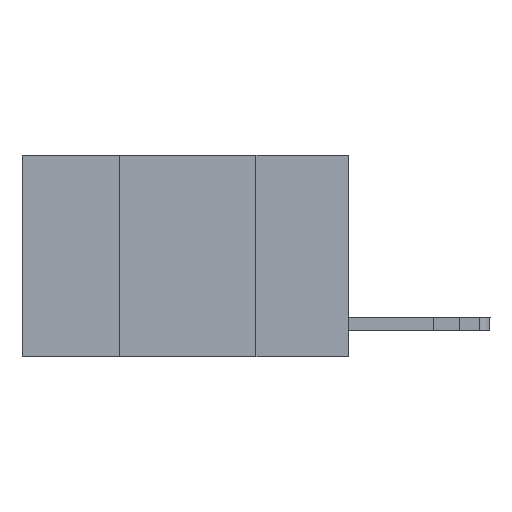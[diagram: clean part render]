
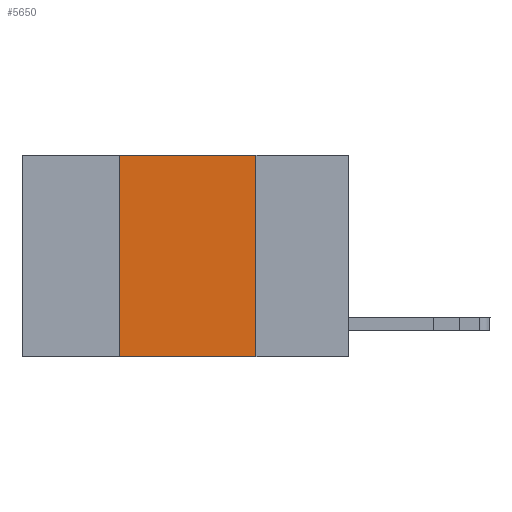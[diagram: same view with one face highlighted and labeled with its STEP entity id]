
A CAD part, left-side view. The second image highlights one B-rep face of the part: STEP entity #5650.
In plain terms, the highlighted planar face has unit normal (-1, 0, 0).
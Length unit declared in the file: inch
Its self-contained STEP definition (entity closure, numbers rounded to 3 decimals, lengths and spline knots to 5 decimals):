
#277 = VECTOR ( 'NONE', #6306, 39.37008 ) ;
#402 = CARTESIAN_POINT ( 'NONE',  ( 0., 0.17, 0. ) ) ;
#588 = VECTOR ( 'NONE', #5456, 39.37008 ) ;
#689 = AXIS2_PLACEMENT_3D ( 'NONE', #2539, #6544, #3451 ) ;
#714 = ORIENTED_EDGE ( 'NONE', *, *, #10044, .F. ) ;
#1664 = PLANE ( 'NONE',  #689 ) ;
#2024 = LINE ( 'NONE', #5980, #6707 ) ;
#2171 = EDGE_CURVE ( 'NONE', #4611, #5207, #12647, .T. ) ;
#2201 = DIRECTION ( 'NONE',  ( 0., -1., 0. ) ) ;
#2539 = CARTESIAN_POINT ( 'NONE',  ( 0., 0.6, 0. ) ) ;
#2913 = EDGE_LOOP ( 'NONE', ( #714, #7543, #7602, #7246 ) ) ;
#3346 = VERTEX_POINT ( 'NONE', #12955 ) ;
#3451 = DIRECTION ( 'NONE',  ( 0., 0., -1. ) ) ;
#4249 = CARTESIAN_POINT ( 'NONE',  ( 0., 0.42, 0. ) ) ;
#4342 = LINE ( 'NONE', #11333, #10923 ) ;
#4425 = CARTESIAN_POINT ( 'NONE',  ( 0., 0.17, -0.37 ) ) ;
#4611 = VERTEX_POINT ( 'NONE', #6180 ) ;
#5207 = VERTEX_POINT ( 'NONE', #4425 ) ;
#5456 = DIRECTION ( 'NONE',  ( 0., -1., 0. ) ) ;
#5650 = ADVANCED_FACE ( 'NONE', ( #12663 ), #1664, .F. ) ;
#5980 = CARTESIAN_POINT ( 'NONE',  ( 0., 0.17, 0. ) ) ;
#6180 = CARTESIAN_POINT ( 'NONE',  ( 0., 0.42, -0.37 ) ) ;
#6306 = DIRECTION ( 'NONE',  ( 0., 0., 1. ) ) ;
#6544 = DIRECTION ( 'NONE',  ( 1., 0., 0. ) ) ;
#6707 = VECTOR ( 'NONE', #12764, 39.37008 ) ;
#7242 = LINE ( 'NONE', #4249, #277 ) ;
#7246 = ORIENTED_EDGE ( 'NONE', *, *, #2171, .T. ) ;
#7300 = VERTEX_POINT ( 'NONE', #402 ) ;
#7543 = ORIENTED_EDGE ( 'NONE', *, *, #8030, .F. ) ;
#7602 = ORIENTED_EDGE ( 'NONE', *, *, #10203, .F. ) ;
#7717 = CARTESIAN_POINT ( 'NONE',  ( 0., 0.6, -0.37 ) ) ;
#8030 = EDGE_CURVE ( 'NONE', #3346, #7300, #4342, .T. ) ;
#10044 = EDGE_CURVE ( 'NONE', #7300, #5207, #2024, .T. ) ;
#10203 = EDGE_CURVE ( 'NONE', #4611, #3346, #7242, .T. ) ;
#10923 = VECTOR ( 'NONE', #2201, 39.37008 ) ;
#11333 = CARTESIAN_POINT ( 'NONE',  ( 0., 0.6, 0. ) ) ;
#12647 = LINE ( 'NONE', #7717, #588 ) ;
#12663 = FACE_OUTER_BOUND ( 'NONE', #2913, .T. ) ;
#12764 = DIRECTION ( 'NONE',  ( 0., 0., -1. ) ) ;
#12955 = CARTESIAN_POINT ( 'NONE',  ( 0., 0.42, 0. ) ) ;
